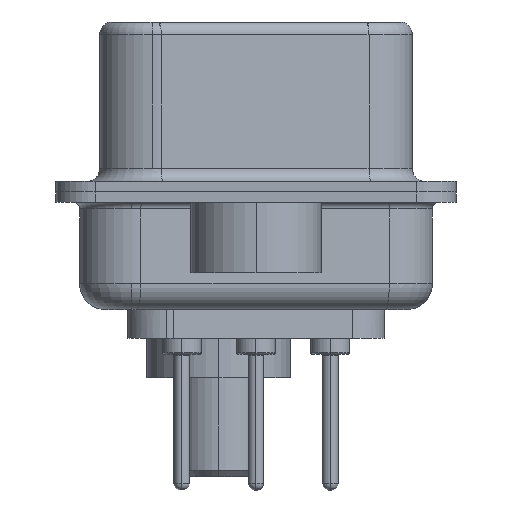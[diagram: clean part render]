
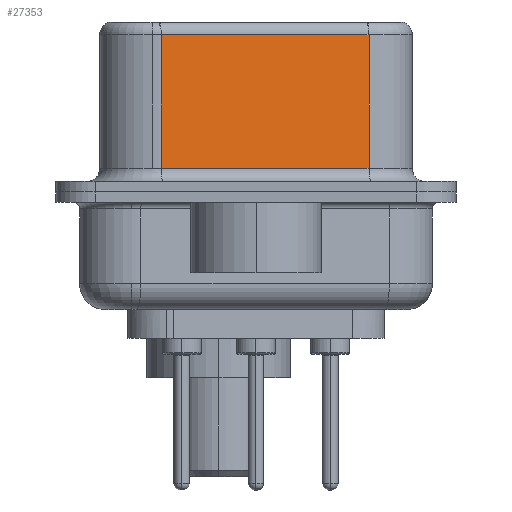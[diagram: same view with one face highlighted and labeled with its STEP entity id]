
A CAD part, left-side view. The second image highlights one B-rep face of the part: STEP entity #27353.
In plain terms, the highlighted planar face has unit normal (-0.985, -0.174, 0).
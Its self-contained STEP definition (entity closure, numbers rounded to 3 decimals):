
#382 = VERTEX_POINT ( 'NONE', #28799 ) ;
#543 = DIRECTION ( 'NONE',  ( 0., 0., -1. ) ) ;
#3590 = LINE ( 'NONE', #24278, #11274 ) ;
#3628 = LINE ( 'NONE', #11517, #20325 ) ;
#4270 = DIRECTION ( 'NONE',  ( 0.985, 0.174, 0. ) ) ;
#5388 = AXIS2_PLACEMENT_3D ( 'NONE', #13567, #4270, #20456 ) ;
#5882 = CARTESIAN_POINT ( 'NONE',  ( 3.73, 3.628, 6.02 ) ) ;
#9879 = VERTEX_POINT ( 'NONE', #16488 ) ;
#11274 = VECTOR ( 'NONE', #15127, 1000. ) ;
#11517 = CARTESIAN_POINT ( 'NONE',  ( 5.132, -4.322, 6.02 ) ) ;
#13177 = CARTESIAN_POINT ( 'NONE',  ( 5.132, -4.322, 0.9 ) ) ;
#13567 = CARTESIAN_POINT ( 'NONE',  ( 5.132, -4.322, 6.52 ) ) ;
#14479 = CARTESIAN_POINT ( 'NONE',  ( 3.73, 3.628, 6.52 ) ) ;
#14533 = ORIENTED_EDGE ( 'NONE', *, *, #19336, .T. ) ;
#15127 = DIRECTION ( 'NONE',  ( 0., 0., -1. ) ) ;
#15215 = LINE ( 'NONE', #13177, #20600 ) ;
#15272 = EDGE_CURVE ( 'NONE', #18428, #27419, #21529, .T. ) ;
#15820 = PLANE ( 'NONE',  #5388 ) ;
#16488 = CARTESIAN_POINT ( 'NONE',  ( 5.132, -4.322, 0.9 ) ) ;
#17697 = FACE_OUTER_BOUND ( 'NONE', #27887, .T. ) ;
#18428 = VERTEX_POINT ( 'NONE', #5882 ) ;
#18432 = CARTESIAN_POINT ( 'NONE',  ( 3.73, 3.628, 0.9 ) ) ;
#19336 = EDGE_CURVE ( 'NONE', #382, #18428, #3628, .T. ) ;
#19690 = ORIENTED_EDGE ( 'NONE', *, *, #27206, .T. ) ;
#20131 = VECTOR ( 'NONE', #543, 1000. ) ;
#20325 = VECTOR ( 'NONE', #22819, 1000. ) ;
#20344 = EDGE_CURVE ( 'NONE', #382, #9879, #3590, .T. ) ;
#20456 = DIRECTION ( 'NONE',  ( -0.174, 0.985, 0. ) ) ;
#20600 = VECTOR ( 'NONE', #29021, 1000. ) ;
#21529 = LINE ( 'NONE', #14479, #20131 ) ;
#22819 = DIRECTION ( 'NONE',  ( -0.174, 0.985, 0. ) ) ;
#24278 = CARTESIAN_POINT ( 'NONE',  ( 5.132, -4.322, 6.52 ) ) ;
#25503 = ORIENTED_EDGE ( 'NONE', *, *, #20344, .F. ) ;
#27206 = EDGE_CURVE ( 'NONE', #27419, #9879, #15215, .T. ) ;
#27353 = ADVANCED_FACE ( 'NONE', ( #17697 ), #15820, .F. ) ;
#27419 = VERTEX_POINT ( 'NONE', #18432 ) ;
#27887 = EDGE_LOOP ( 'NONE', ( #25503, #14533, #28558, #19690 ) ) ;
#28558 = ORIENTED_EDGE ( 'NONE', *, *, #15272, .T. ) ;
#28799 = CARTESIAN_POINT ( 'NONE',  ( 5.132, -4.322, 6.02 ) ) ;
#29021 = DIRECTION ( 'NONE',  ( 0.174, -0.985, 0. ) ) ;
